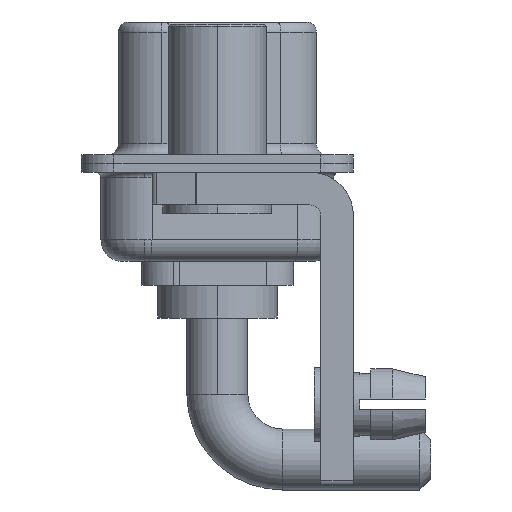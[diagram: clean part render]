
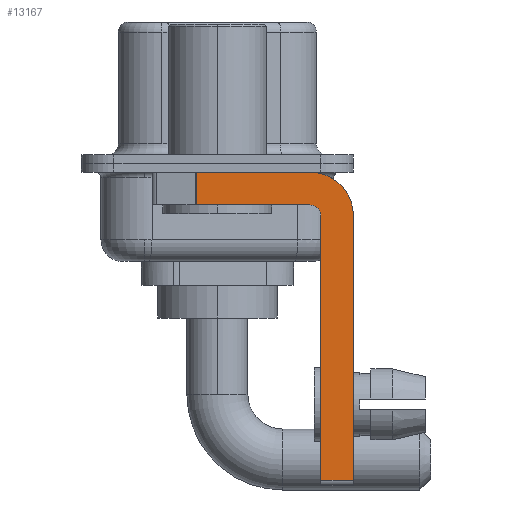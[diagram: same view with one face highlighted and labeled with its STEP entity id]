
A CAD part, left-side view. The second image highlights one B-rep face of the part: STEP entity #13167.
In plain terms, the highlighted planar face has unit normal (-1, 0, 0).
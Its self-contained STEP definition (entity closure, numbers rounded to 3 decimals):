
#70 = CARTESIAN_POINT ( 'NONE',  ( -2.9, -4.25, -2.4 ) ) ;
#86 = CARTESIAN_POINT ( 'NONE',  ( -2.9, -6.25, -2.4 ) ) ;
#159 = VERTEX_POINT ( 'NONE', #6272 ) ;
#291 = CARTESIAN_POINT ( 'NONE',  ( -2.9, -4.75, -2.4 ) ) ;
#454 = EDGE_CURVE ( 'NONE', #8944, #9301, #6980, .T. ) ;
#1086 = EDGE_LOOP ( 'NONE', ( #15635, #10216, #8729, #5256, #10298, #2831, #7814, #8501 ) ) ;
#1438 = DIRECTION ( 'NONE',  ( 0., 0., 1. ) ) ;
#2154 = DIRECTION ( 'NONE',  ( 0., 0., -1. ) ) ;
#2357 = VERTEX_POINT ( 'NONE', #12860 ) ;
#2649 = DIRECTION ( 'NONE',  ( 1., 0., 0. ) ) ;
#2831 = ORIENTED_EDGE ( 'NONE', *, *, #11073, .T. ) ;
#2889 = CARTESIAN_POINT ( 'NONE',  ( -2.9, -6.25, -2.4 ) ) ;
#3206 = VECTOR ( 'NONE', #14316, 1000. ) ;
#4664 = EDGE_CURVE ( 'NONE', #8721, #8944, #15302, .T. ) ;
#4884 = EDGE_CURVE ( 'NONE', #2357, #8721, #13674, .T. ) ;
#4938 = DIRECTION ( 'NONE',  ( 0., 0., 1. ) ) ;
#4993 = VECTOR ( 'NONE', #12606, 1000. ) ;
#5004 = DIRECTION ( 'NONE',  ( 0., -1., 0. ) ) ;
#5108 = CARTESIAN_POINT ( 'NONE',  ( -2.9, 0.978, -1.9 ) ) ;
#5144 = EDGE_CURVE ( 'NONE', #13894, #5892, #7672, .T. ) ;
#5256 = ORIENTED_EDGE ( 'NONE', *, *, #12395, .F. ) ;
#5744 = EDGE_CURVE ( 'NONE', #2357, #13200, #15734, .T. ) ;
#5892 = VERTEX_POINT ( 'NONE', #291 ) ;
#6054 = CARTESIAN_POINT ( 'NONE',  ( -2.9, -4.75, -14.55 ) ) ;
#6272 = CARTESIAN_POINT ( 'NONE',  ( -2.9, -4.25, -1.9 ) ) ;
#6420 = CARTESIAN_POINT ( 'NONE',  ( -2.9, -4.25, -2.4 ) ) ;
#6980 = LINE ( 'NONE', #86, #4993 ) ;
#7004 = CIRCLE ( 'NONE', #9599, 0.5 ) ;
#7672 = LINE ( 'NONE', #14390, #13017 ) ;
#7790 = VECTOR ( 'NONE', #7859, 1000. ) ;
#7814 = ORIENTED_EDGE ( 'NONE', *, *, #454, .F. ) ;
#7859 = DIRECTION ( 'NONE',  ( 0., -1., 0. ) ) ;
#8037 = CARTESIAN_POINT ( 'NONE',  ( -2.9, 3., -0.4 ) ) ;
#8501 = ORIENTED_EDGE ( 'NONE', *, *, #4664, .F. ) ;
#8721 = VERTEX_POINT ( 'NONE', #11364 ) ;
#8729 = ORIENTED_EDGE ( 'NONE', *, *, #9082, .F. ) ;
#8944 = VERTEX_POINT ( 'NONE', #2889 ) ;
#9082 = EDGE_CURVE ( 'NONE', #159, #13200, #14412, .T. ) ;
#9301 = VERTEX_POINT ( 'NONE', #10931 ) ;
#9460 = FACE_OUTER_BOUND ( 'NONE', #1086, .T. ) ;
#9537 = CARTESIAN_POINT ( 'NONE',  ( -2.9, -4.25, -14.55 ) ) ;
#9599 = AXIS2_PLACEMENT_3D ( 'NONE', #70, #13956, #1438 ) ;
#10216 = ORIENTED_EDGE ( 'NONE', *, *, #5744, .T. ) ;
#10298 = ORIENTED_EDGE ( 'NONE', *, *, #5144, .F. ) ;
#10777 = AXIS2_PLACEMENT_3D ( 'NONE', #11996, #2649, #12086 ) ;
#10931 = CARTESIAN_POINT ( 'NONE',  ( -2.9, -6.25, -14.55 ) ) ;
#11073 = EDGE_CURVE ( 'NONE', #13894, #9301, #12253, .T. ) ;
#11364 = CARTESIAN_POINT ( 'NONE',  ( -2.9, -4.25, -0.4 ) ) ;
#11678 = DIRECTION ( 'NONE',  ( 1., 0., 0. ) ) ;
#11996 = CARTESIAN_POINT ( 'NONE',  ( -2.9, -4.25, -2.4 ) ) ;
#12086 = DIRECTION ( 'NONE',  ( 0., 0., -1. ) ) ;
#12104 = AXIS2_PLACEMENT_3D ( 'NONE', #6420, #11678, #2154 ) ;
#12253 = LINE ( 'NONE', #9537, #14437 ) ;
#12395 = EDGE_CURVE ( 'NONE', #5892, #159, #7004, .T. ) ;
#12606 = DIRECTION ( 'NONE',  ( 0., 0., -1. ) ) ;
#12860 = CARTESIAN_POINT ( 'NONE',  ( -2.9, 0.978, -0.4 ) ) ;
#13017 = VECTOR ( 'NONE', #4938, 1000. ) ;
#13167 = ADVANCED_FACE ( 'NONE', ( #9460 ), #16359, .F. ) ;
#13200 = VERTEX_POINT ( 'NONE', #5108 ) ;
#13309 = VECTOR ( 'NONE', #16348, 1000. ) ;
#13674 = LINE ( 'NONE', #8037, #7790 ) ;
#13894 = VERTEX_POINT ( 'NONE', #6054 ) ;
#13956 = DIRECTION ( 'NONE',  ( -1., 0., 0. ) ) ;
#14316 = DIRECTION ( 'NONE',  ( 0., 1., 0. ) ) ;
#14390 = CARTESIAN_POINT ( 'NONE',  ( -2.9, -4.75, -14.8 ) ) ;
#14412 = LINE ( 'NONE', #14496, #3206 ) ;
#14437 = VECTOR ( 'NONE', #5004, 1000. ) ;
#14496 = CARTESIAN_POINT ( 'NONE',  ( -2.9, -4.25, -1.9 ) ) ;
#15302 = CIRCLE ( 'NONE', #12104, 2. ) ;
#15635 = ORIENTED_EDGE ( 'NONE', *, *, #4884, .F. ) ;
#15734 = LINE ( 'NONE', #16091, #13309 ) ;
#16091 = CARTESIAN_POINT ( 'NONE',  ( -2.9, 0.978, -1.9 ) ) ;
#16348 = DIRECTION ( 'NONE',  ( 0., 0., -1. ) ) ;
#16359 = PLANE ( 'NONE',  #10777 ) ;
